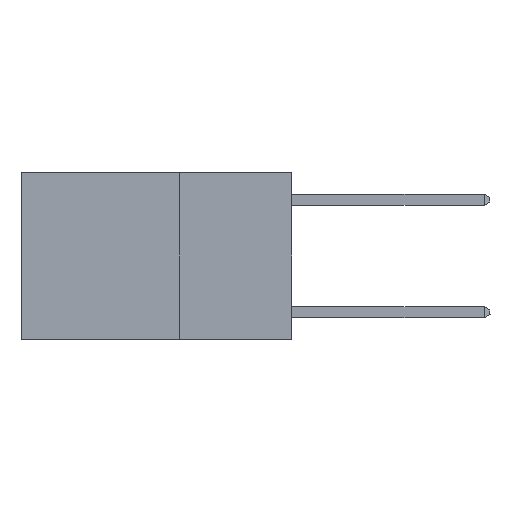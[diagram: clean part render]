
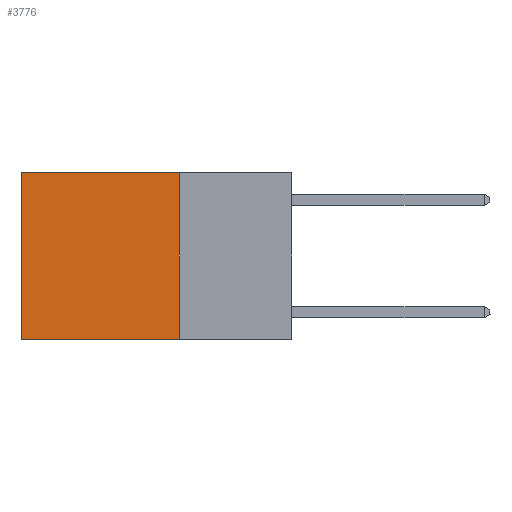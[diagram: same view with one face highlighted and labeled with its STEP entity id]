
A CAD part, left-side view. The second image highlights one B-rep face of the part: STEP entity #3776.
In plain terms, the highlighted planar face has unit normal (-1, 0, 0).
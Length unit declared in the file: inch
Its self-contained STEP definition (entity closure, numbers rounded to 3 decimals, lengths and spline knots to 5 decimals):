
#1337 = LINE ( 'NONE', #25613, #17113 ) ;
#2330 = DIRECTION ( 'NONE',  ( 0., 0., -1. ) ) ;
#2580 = DIRECTION ( 'NONE',  ( 0., 0., -1. ) ) ;
#2607 = LINE ( 'NONE', #14650, #9566 ) ;
#3776 = ADVANCED_FACE ( 'NONE', ( #8762 ), #25491, .F. ) ;
#4589 = EDGE_CURVE ( 'NONE', #24635, #4993, #8665, .T. ) ;
#4993 = VERTEX_POINT ( 'NONE', #10743 ) ;
#5238 = DIRECTION ( 'NONE',  ( 0., 0., -1. ) ) ;
#5348 = CARTESIAN_POINT ( 'NONE',  ( 0.2625, 0.25, -0.37 ) ) ;
#6383 = VERTEX_POINT ( 'NONE', #20872 ) ;
#6388 = EDGE_CURVE ( 'NONE', #6383, #24635, #12508, .T. ) ;
#6514 = DIRECTION ( 'NONE',  ( 0., 1., 0. ) ) ;
#6732 = ORIENTED_EDGE ( 'NONE', *, *, #4589, .F. ) ;
#8433 = ORIENTED_EDGE ( 'NONE', *, *, #14881, .T. ) ;
#8665 = LINE ( 'NONE', #14659, #16995 ) ;
#8683 = CARTESIAN_POINT ( 'NONE',  ( 0.2625, 0.6, 0. ) ) ;
#8762 = FACE_OUTER_BOUND ( 'NONE', #11695, .T. ) ;
#9566 = VECTOR ( 'NONE', #18506, 39.37008 ) ;
#9652 = ORIENTED_EDGE ( 'NONE', *, *, #6388, .F. ) ;
#10743 = CARTESIAN_POINT ( 'NONE',  ( 0.2625, 0.6, -0.37 ) ) ;
#11695 = EDGE_LOOP ( 'NONE', ( #23226, #6732, #9652, #8433 ) ) ;
#12508 = LINE ( 'NONE', #20616, #23339 ) ;
#13250 = AXIS2_PLACEMENT_3D ( 'NONE', #22993, #19253, #2580 ) ;
#14650 = CARTESIAN_POINT ( 'NONE',  ( 0.2625, 0.25, 0. ) ) ;
#14659 = CARTESIAN_POINT ( 'NONE',  ( 0.2625, 0.25, -0.37 ) ) ;
#14881 = EDGE_CURVE ( 'NONE', #6383, #24872, #2607, .T. ) ;
#16995 = VECTOR ( 'NONE', #6514, 39.37008 ) ;
#17113 = VECTOR ( 'NONE', #5238, 39.37008 ) ;
#18506 = DIRECTION ( 'NONE',  ( 0., 1., 0. ) ) ;
#19253 = DIRECTION ( 'NONE',  ( 1., 0., 0. ) ) ;
#20616 = CARTESIAN_POINT ( 'NONE',  ( 0.2625, 0.25, 0. ) ) ;
#20872 = CARTESIAN_POINT ( 'NONE',  ( 0.2625, 0.25, 0. ) ) ;
#22993 = CARTESIAN_POINT ( 'NONE',  ( 0.2625, 0.25, 0. ) ) ;
#23226 = ORIENTED_EDGE ( 'NONE', *, *, #24147, .T. ) ;
#23339 = VECTOR ( 'NONE', #2330, 39.37008 ) ;
#24147 = EDGE_CURVE ( 'NONE', #24872, #4993, #1337, .T. ) ;
#24635 = VERTEX_POINT ( 'NONE', #5348 ) ;
#24872 = VERTEX_POINT ( 'NONE', #8683 ) ;
#25491 = PLANE ( 'NONE',  #13250 ) ;
#25613 = CARTESIAN_POINT ( 'NONE',  ( 0.2625, 0.6, 0. ) ) ;
